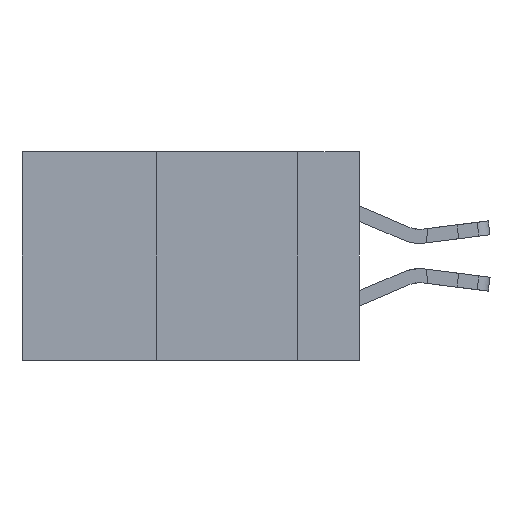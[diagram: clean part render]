
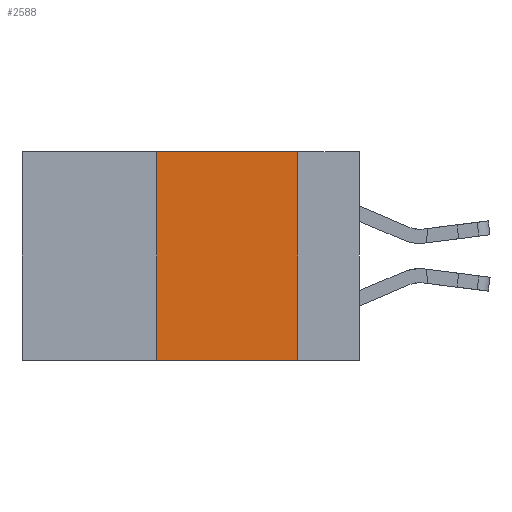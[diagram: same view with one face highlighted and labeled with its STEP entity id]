
A CAD part, left-side view. The second image highlights one B-rep face of the part: STEP entity #2588.
In plain terms, the highlighted planar face has unit normal (-1, 0, 0).
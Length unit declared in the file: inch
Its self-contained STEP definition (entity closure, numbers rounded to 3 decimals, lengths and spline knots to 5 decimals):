
#2588 = ADVANCED_FACE ( 'NONE', ( #18114 ), #20016, .F. ) ;
#4005 = ORIENTED_EDGE ( 'NONE', *, *, #33775, .F. ) ;
#4254 = DIRECTION ( 'NONE',  ( 0., 0., -1. ) ) ;
#5569 = LINE ( 'NONE', #10747, #11464 ) ;
#6108 = VERTEX_POINT ( 'NONE', #9731 ) ;
#7026 = VECTOR ( 'NONE', #20504, 39.37008 ) ;
#9731 = CARTESIAN_POINT ( 'NONE',  ( 0., 0.36, 0. ) ) ;
#10385 = LINE ( 'NONE', #20790, #31245 ) ;
#10435 = CARTESIAN_POINT ( 'NONE',  ( 0., 0.6, -0.37 ) ) ;
#10747 = CARTESIAN_POINT ( 'NONE',  ( 0., 0.11, 0. ) ) ;
#11464 = VECTOR ( 'NONE', #16073, 39.37008 ) ;
#11623 = EDGE_LOOP ( 'NONE', ( #4005, #27417, #23163, #13242 ) ) ;
#11649 = EDGE_CURVE ( 'NONE', #14975, #6108, #10385, .T. ) ;
#13242 = ORIENTED_EDGE ( 'NONE', *, *, #30284, .T. ) ;
#14975 = VERTEX_POINT ( 'NONE', #30297 ) ;
#15120 = CARTESIAN_POINT ( 'NONE',  ( 0., 0.6, 0. ) ) ;
#15790 = DIRECTION ( 'NONE',  ( 0., -1., 0. ) ) ;
#16073 = DIRECTION ( 'NONE',  ( 0., 0., -1. ) ) ;
#16507 = VECTOR ( 'NONE', #15790, 39.37008 ) ;
#16991 = LINE ( 'NONE', #31134, #7026 ) ;
#17302 = AXIS2_PLACEMENT_3D ( 'NONE', #15120, #31118, #4254 ) ;
#17743 = LINE ( 'NONE', #10435, #16507 ) ;
#18114 = FACE_OUTER_BOUND ( 'NONE', #11623, .T. ) ;
#18827 = CARTESIAN_POINT ( 'NONE',  ( 0., 0.11, -0.37 ) ) ;
#20016 = PLANE ( 'NONE',  #17302 ) ;
#20504 = DIRECTION ( 'NONE',  ( 0., -1., 0. ) ) ;
#20790 = CARTESIAN_POINT ( 'NONE',  ( 0., 0.36, 0. ) ) ;
#22147 = VERTEX_POINT ( 'NONE', #18827 ) ;
#23163 = ORIENTED_EDGE ( 'NONE', *, *, #11649, .F. ) ;
#27417 = ORIENTED_EDGE ( 'NONE', *, *, #31530, .F. ) ;
#28852 = DIRECTION ( 'NONE',  ( 0., 0., 1. ) ) ;
#30284 = EDGE_CURVE ( 'NONE', #14975, #22147, #17743, .T. ) ;
#30297 = CARTESIAN_POINT ( 'NONE',  ( 0., 0.36, -0.37 ) ) ;
#30637 = CARTESIAN_POINT ( 'NONE',  ( 0., 0.11, 0. ) ) ;
#31118 = DIRECTION ( 'NONE',  ( 1., 0., 0. ) ) ;
#31134 = CARTESIAN_POINT ( 'NONE',  ( 0., 0.6, 0. ) ) ;
#31245 = VECTOR ( 'NONE', #28852, 39.37008 ) ;
#31530 = EDGE_CURVE ( 'NONE', #6108, #32836, #16991, .T. ) ;
#32836 = VERTEX_POINT ( 'NONE', #30637 ) ;
#33775 = EDGE_CURVE ( 'NONE', #32836, #22147, #5569, .T. ) ;
